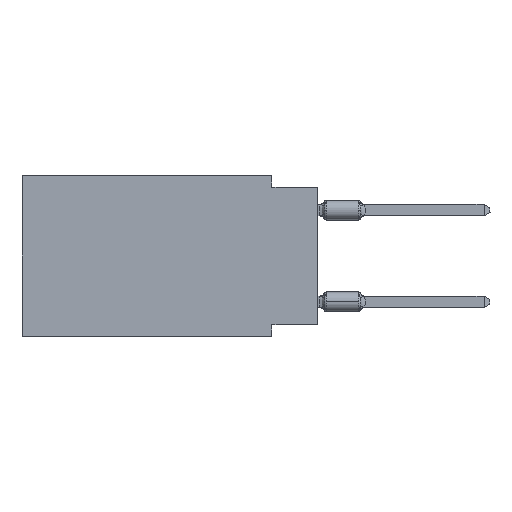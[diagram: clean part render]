
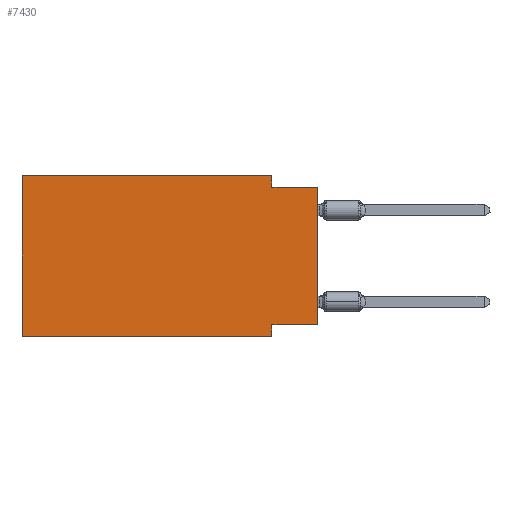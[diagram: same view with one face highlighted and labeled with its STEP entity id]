
A CAD part, left-side view. The second image highlights one B-rep face of the part: STEP entity #7430.
In plain terms, the highlighted planar face has unit normal (-1, 0, 0).
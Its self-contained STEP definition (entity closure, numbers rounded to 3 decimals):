
#686 = FACE_OUTER_BOUND ( 'NONE', #21618, .T. ) ;
#975 = CARTESIAN_POINT ( 'NONE',  ( 0., 2.54, 0. ) ) ;
#2119 = VECTOR ( 'NONE', #5237, 1000. ) ;
#2638 = DIRECTION ( 'NONE',  ( 0., -1., 0. ) ) ;
#3478 = ORIENTED_EDGE ( 'NONE', *, *, #6723, .F. ) ;
#4109 = EDGE_CURVE ( 'NONE', #13061, #37529, #25266, .T. ) ;
#4275 = VERTEX_POINT ( 'NONE', #39747 ) ;
#4682 = EDGE_CURVE ( 'NONE', #7679, #13061, #19766, .T. ) ;
#5237 = DIRECTION ( 'NONE',  ( 0., -1., 0. ) ) ;
#5242 = CARTESIAN_POINT ( 'NONE',  ( 0., 2.54, -0.635 ) ) ;
#5860 = VERTEX_POINT ( 'NONE', #25638 ) ;
#6348 = CARTESIAN_POINT ( 'NONE',  ( 0., 2.54, -8.255 ) ) ;
#6659 = ORIENTED_EDGE ( 'NONE', *, *, #4109, .F. ) ;
#6723 = EDGE_CURVE ( 'NONE', #37561, #7679, #7988, .T. ) ;
#7430 = ADVANCED_FACE ( 'NONE', ( #686 ), #10647, .F. ) ;
#7679 = VERTEX_POINT ( 'NONE', #14273 ) ;
#7988 = LINE ( 'NONE', #14920, #28174 ) ;
#8245 = DIRECTION ( 'NONE',  ( 0., 0., -1. ) ) ;
#9350 = CARTESIAN_POINT ( 'NONE',  ( 0., 16.383, -8.89 ) ) ;
#9504 = EDGE_CURVE ( 'NONE', #16838, #4275, #31117, .T. ) ;
#9522 = AXIS2_PLACEMENT_3D ( 'NONE', #37096, #20636, #8245 ) ;
#9659 = VECTOR ( 'NONE', #30695, 1000. ) ;
#10030 = LINE ( 'NONE', #29987, #17130 ) ;
#10647 = PLANE ( 'NONE',  #9522 ) ;
#11814 = VECTOR ( 'NONE', #28849, 1000. ) ;
#12504 = CARTESIAN_POINT ( 'NONE',  ( 0., 0., 0. ) ) ;
#13061 = VERTEX_POINT ( 'NONE', #975 ) ;
#14020 = CARTESIAN_POINT ( 'NONE',  ( 0., 2.54, -8.89 ) ) ;
#14273 = CARTESIAN_POINT ( 'NONE',  ( 0., 16.383, 0. ) ) ;
#14795 = EDGE_CURVE ( 'NONE', #37561, #4275, #18470, .T. ) ;
#14920 = CARTESIAN_POINT ( 'NONE',  ( 0., 16.383, 0. ) ) ;
#16548 = VECTOR ( 'NONE', #28563, 1000. ) ;
#16838 = VERTEX_POINT ( 'NONE', #6348 ) ;
#17130 = VECTOR ( 'NONE', #42793, 1000. ) ;
#18016 = CARTESIAN_POINT ( 'NONE',  ( 0., 0., -0.635 ) ) ;
#18470 = LINE ( 'NONE', #29296, #2119 ) ;
#19160 = EDGE_CURVE ( 'NONE', #5860, #28891, #35262, .T. ) ;
#19766 = LINE ( 'NONE', #38852, #32553 ) ;
#20636 = DIRECTION ( 'NONE',  ( 1., 0., 0. ) ) ;
#20808 = VECTOR ( 'NONE', #31741, 1000. ) ;
#21401 = EDGE_CURVE ( 'NONE', #5860, #16838, #41232, .T. ) ;
#21618 = EDGE_LOOP ( 'NONE', ( #22113, #40533, #6659, #35386, #3478, #28736, #33803, #27750 ) ) ;
#22113 = ORIENTED_EDGE ( 'NONE', *, *, #19160, .T. ) ;
#25266 = LINE ( 'NONE', #42167, #20808 ) ;
#25638 = CARTESIAN_POINT ( 'NONE',  ( 0., 0., -8.255 ) ) ;
#27750 = ORIENTED_EDGE ( 'NONE', *, *, #21401, .F. ) ;
#28174 = VECTOR ( 'NONE', #34408, 1000. ) ;
#28434 = CARTESIAN_POINT ( 'NONE',  ( 0., 0., -8.255 ) ) ;
#28563 = DIRECTION ( 'NONE',  ( 0., 0., 1. ) ) ;
#28736 = ORIENTED_EDGE ( 'NONE', *, *, #14795, .T. ) ;
#28849 = DIRECTION ( 'NONE',  ( 0., 1., 0. ) ) ;
#28891 = VERTEX_POINT ( 'NONE', #18016 ) ;
#29296 = CARTESIAN_POINT ( 'NONE',  ( 0., 16.383, -8.89 ) ) ;
#29987 = CARTESIAN_POINT ( 'NONE',  ( 0., 0., -0.635 ) ) ;
#30695 = DIRECTION ( 'NONE',  ( 0., 0., -1. ) ) ;
#31117 = LINE ( 'NONE', #14020, #9659 ) ;
#31741 = DIRECTION ( 'NONE',  ( 0., 0., -1. ) ) ;
#31949 = EDGE_CURVE ( 'NONE', #37529, #28891, #10030, .T. ) ;
#32553 = VECTOR ( 'NONE', #2638, 1000. ) ;
#33803 = ORIENTED_EDGE ( 'NONE', *, *, #9504, .F. ) ;
#34408 = DIRECTION ( 'NONE',  ( 0., 0., 1. ) ) ;
#35262 = LINE ( 'NONE', #12504, #16548 ) ;
#35386 = ORIENTED_EDGE ( 'NONE', *, *, #4682, .F. ) ;
#37096 = CARTESIAN_POINT ( 'NONE',  ( 0., 16.383, 0. ) ) ;
#37529 = VERTEX_POINT ( 'NONE', #5242 ) ;
#37561 = VERTEX_POINT ( 'NONE', #9350 ) ;
#38852 = CARTESIAN_POINT ( 'NONE',  ( 0., 16.383, 0. ) ) ;
#39747 = CARTESIAN_POINT ( 'NONE',  ( 0., 2.54, -8.89 ) ) ;
#40533 = ORIENTED_EDGE ( 'NONE', *, *, #31949, .F. ) ;
#41232 = LINE ( 'NONE', #28434, #11814 ) ;
#42167 = CARTESIAN_POINT ( 'NONE',  ( 0., 2.54, 0. ) ) ;
#42793 = DIRECTION ( 'NONE',  ( 0., -1., 0. ) ) ;
